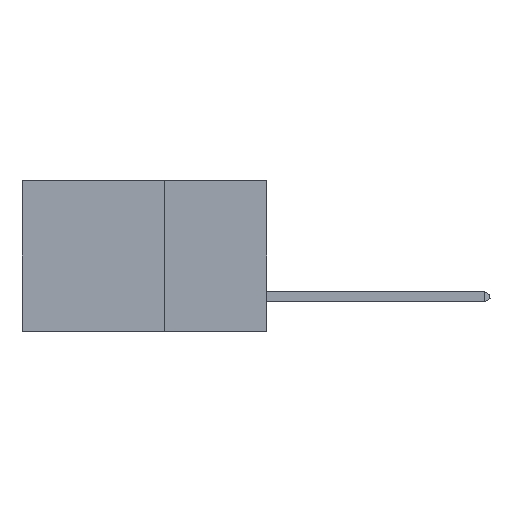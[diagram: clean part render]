
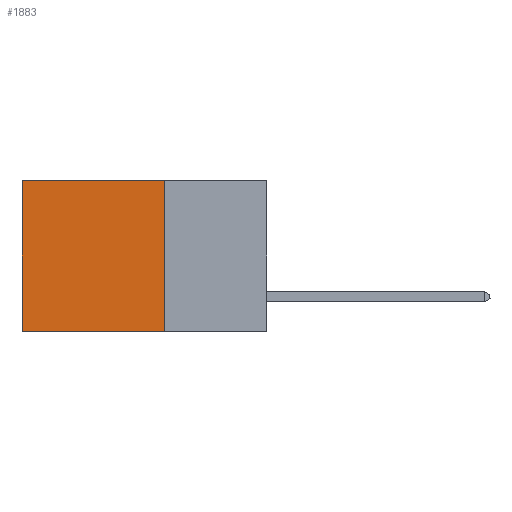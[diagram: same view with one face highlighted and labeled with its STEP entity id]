
A CAD part, left-side view. The second image highlights one B-rep face of the part: STEP entity #1883.
In plain terms, the highlighted planar face has unit normal (-1, 0, 0).
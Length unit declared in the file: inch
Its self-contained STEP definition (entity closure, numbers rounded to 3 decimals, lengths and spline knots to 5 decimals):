
#332 = EDGE_CURVE ( 'NONE', #11502, #16010, #7173, .T. ) ;
#399 = CARTESIAN_POINT ( 'NONE',  ( 0.2875, 0.25, 0. ) ) ;
#868 = ORIENTED_EDGE ( 'NONE', *, *, #17623, .T. ) ;
#1258 = DIRECTION ( 'NONE',  ( 0., 0., -1. ) ) ;
#1269 = DIRECTION ( 'NONE',  ( 0., 1., 0. ) ) ;
#1355 = LINE ( 'NONE', #11423, #17165 ) ;
#1883 = ADVANCED_FACE ( 'NONE', ( #6000 ), #4018, .F. ) ;
#2608 = CARTESIAN_POINT ( 'NONE',  ( 0.2875, 0.6, -0.37 ) ) ;
#2833 = VERTEX_POINT ( 'NONE', #6823 ) ;
#3559 = VECTOR ( 'NONE', #1269, 39.37008 ) ;
#4018 = PLANE ( 'NONE',  #12010 ) ;
#5008 = LINE ( 'NONE', #18087, #19634 ) ;
#5531 = CARTESIAN_POINT ( 'NONE',  ( 0.2875, 0.25, -0.37 ) ) ;
#5789 = CARTESIAN_POINT ( 'NONE',  ( 0.2875, 0.25, -0.37 ) ) ;
#6000 = FACE_OUTER_BOUND ( 'NONE', #12207, .T. ) ;
#6126 = EDGE_CURVE ( 'NONE', #2833, #15401, #14200, .T. ) ;
#6539 = VECTOR ( 'NONE', #8117, 39.37008 ) ;
#6823 = CARTESIAN_POINT ( 'NONE',  ( 0.2875, 0.25, 0. ) ) ;
#6968 = DIRECTION ( 'NONE',  ( 1., 0., 0. ) ) ;
#7099 = CARTESIAN_POINT ( 'NONE',  ( 0.2875, 0.25, 0. ) ) ;
#7173 = LINE ( 'NONE', #5789, #3559 ) ;
#8117 = DIRECTION ( 'NONE',  ( 0., 1., 0. ) ) ;
#11423 = CARTESIAN_POINT ( 'NONE',  ( 0.2875, 0.6, 0. ) ) ;
#11502 = VERTEX_POINT ( 'NONE', #5531 ) ;
#11664 = ORIENTED_EDGE ( 'NONE', *, *, #332, .F. ) ;
#12010 = AXIS2_PLACEMENT_3D ( 'NONE', #7099, #6968, #17613 ) ;
#12207 = EDGE_LOOP ( 'NONE', ( #868, #11664, #18898, #13924 ) ) ;
#13924 = ORIENTED_EDGE ( 'NONE', *, *, #6126, .T. ) ;
#14200 = LINE ( 'NONE', #399, #6539 ) ;
#14621 = CARTESIAN_POINT ( 'NONE',  ( 0.2875, 0.6, 0. ) ) ;
#15401 = VERTEX_POINT ( 'NONE', #14621 ) ;
#16010 = VERTEX_POINT ( 'NONE', #2608 ) ;
#16762 = EDGE_CURVE ( 'NONE', #2833, #11502, #5008, .T. ) ;
#17165 = VECTOR ( 'NONE', #17301, 39.37008 ) ;
#17301 = DIRECTION ( 'NONE',  ( 0., 0., -1. ) ) ;
#17613 = DIRECTION ( 'NONE',  ( 0., 0., -1. ) ) ;
#17623 = EDGE_CURVE ( 'NONE', #15401, #16010, #1355, .T. ) ;
#18087 = CARTESIAN_POINT ( 'NONE',  ( 0.2875, 0.25, 0. ) ) ;
#18898 = ORIENTED_EDGE ( 'NONE', *, *, #16762, .F. ) ;
#19634 = VECTOR ( 'NONE', #1258, 39.37008 ) ;
